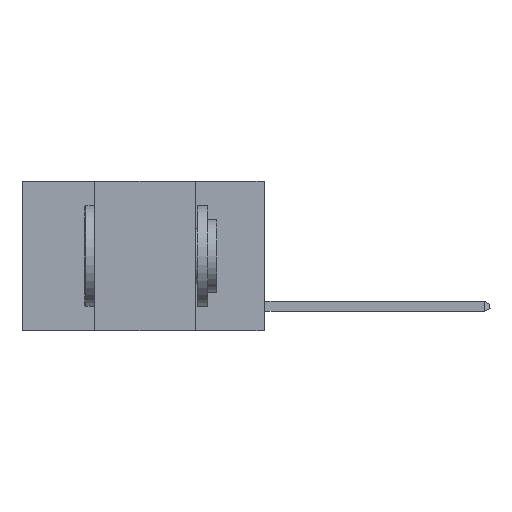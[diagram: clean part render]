
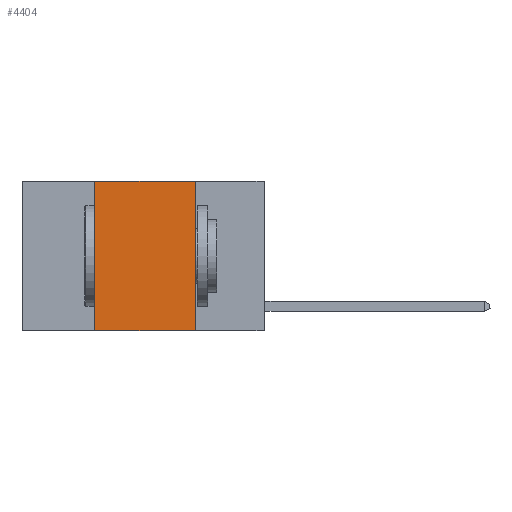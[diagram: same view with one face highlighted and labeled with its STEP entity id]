
A CAD part, left-side view. The second image highlights one B-rep face of the part: STEP entity #4404.
In plain terms, the highlighted planar face has unit normal (-1, 0, 0).
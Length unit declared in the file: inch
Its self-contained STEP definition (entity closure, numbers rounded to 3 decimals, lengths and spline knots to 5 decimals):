
#551 = EDGE_LOOP ( 'NONE', ( #1624, #7836, #8245, #6836 ) ) ;
#642 = PLANE ( 'NONE',  #8819 ) ;
#950 = VERTEX_POINT ( 'NONE', #4071 ) ;
#1355 = CARTESIAN_POINT ( 'NONE',  ( 0., 0.6, 0. ) ) ;
#1419 = CARTESIAN_POINT ( 'NONE',  ( 0., 0.6, -0.37 ) ) ;
#1473 = DIRECTION ( 'NONE',  ( 1., 0., 0. ) ) ;
#1624 = ORIENTED_EDGE ( 'NONE', *, *, #7620, .F. ) ;
#1724 = EDGE_CURVE ( 'NONE', #8618, #2008, #4082, .T. ) ;
#2008 = VERTEX_POINT ( 'NONE', #9224 ) ;
#2411 = EDGE_CURVE ( 'NONE', #5822, #8618, #11656, .T. ) ;
#2624 = DIRECTION ( 'NONE',  ( 0., 0., 1. ) ) ;
#3011 = CARTESIAN_POINT ( 'NONE',  ( 0., 0.42, 0. ) ) ;
#4071 = CARTESIAN_POINT ( 'NONE',  ( 0., 0.17, -0.37 ) ) ;
#4082 = LINE ( 'NONE', #7692, #7053 ) ;
#4404 = ADVANCED_FACE ( 'NONE', ( #5963 ), #642, .F. ) ;
#4487 = LINE ( 'NONE', #10837, #7147 ) ;
#5763 = CARTESIAN_POINT ( 'NONE',  ( 0., 0.42, -0.37 ) ) ;
#5822 = VERTEX_POINT ( 'NONE', #5763 ) ;
#5892 = DIRECTION ( 'NONE',  ( 0., -1., 0. ) ) ;
#5963 = FACE_OUTER_BOUND ( 'NONE', #551, .T. ) ;
#6680 = VECTOR ( 'NONE', #2624, 39.37008 ) ;
#6836 = ORIENTED_EDGE ( 'NONE', *, *, #8169, .T. ) ;
#7053 = VECTOR ( 'NONE', #5892, 39.37008 ) ;
#7135 = CARTESIAN_POINT ( 'NONE',  ( 0., 0.42, 0. ) ) ;
#7147 = VECTOR ( 'NONE', #7282, 39.37008 ) ;
#7282 = DIRECTION ( 'NONE',  ( 0., 0., -1. ) ) ;
#7620 = EDGE_CURVE ( 'NONE', #2008, #950, #4487, .T. ) ;
#7692 = CARTESIAN_POINT ( 'NONE',  ( 0., 0.6, 0. ) ) ;
#7836 = ORIENTED_EDGE ( 'NONE', *, *, #1724, .F. ) ;
#7908 = VECTOR ( 'NONE', #9376, 39.37008 ) ;
#8169 = EDGE_CURVE ( 'NONE', #5822, #950, #10390, .T. ) ;
#8245 = ORIENTED_EDGE ( 'NONE', *, *, #2411, .F. ) ;
#8618 = VERTEX_POINT ( 'NONE', #3011 ) ;
#8819 = AXIS2_PLACEMENT_3D ( 'NONE', #1355, #1473, #9553 ) ;
#9224 = CARTESIAN_POINT ( 'NONE',  ( 0., 0.17, 0. ) ) ;
#9376 = DIRECTION ( 'NONE',  ( 0., -1., 0. ) ) ;
#9553 = DIRECTION ( 'NONE',  ( 0., 0., -1. ) ) ;
#10390 = LINE ( 'NONE', #1419, #7908 ) ;
#10837 = CARTESIAN_POINT ( 'NONE',  ( 0., 0.17, 0. ) ) ;
#11656 = LINE ( 'NONE', #7135, #6680 ) ;
